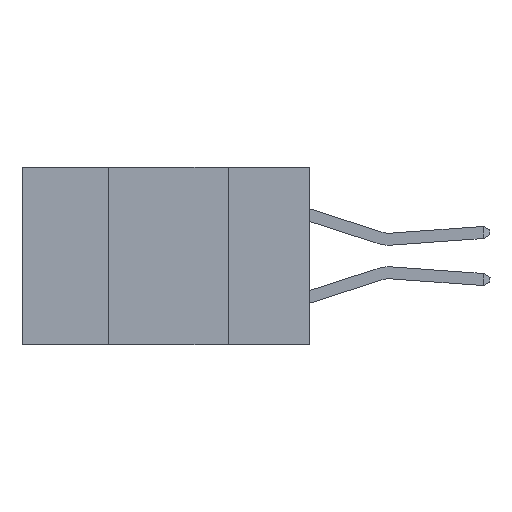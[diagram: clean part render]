
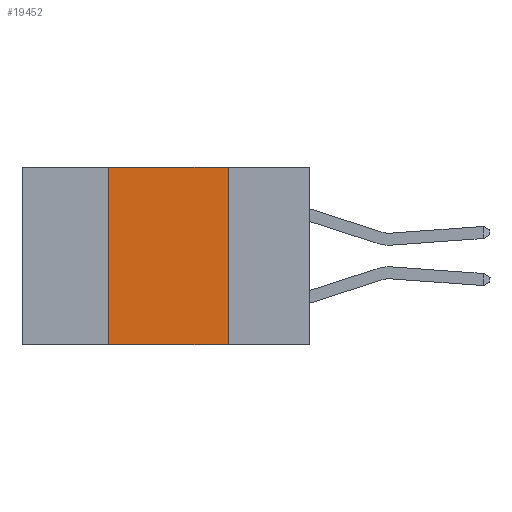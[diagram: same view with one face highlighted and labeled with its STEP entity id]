
A CAD part, left-side view. The second image highlights one B-rep face of the part: STEP entity #19452.
In plain terms, the highlighted planar face has unit normal (-1, 0, 0).
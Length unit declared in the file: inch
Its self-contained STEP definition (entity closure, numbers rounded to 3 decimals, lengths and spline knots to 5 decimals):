
#241 = FACE_OUTER_BOUND ( 'NONE', #21795, .T. ) ;
#1564 = EDGE_CURVE ( 'NONE', #21001, #3537, #8255, .T. ) ;
#2190 = DIRECTION ( 'NONE',  ( 0., -1., 0. ) ) ;
#2445 = DIRECTION ( 'NONE',  ( 0., 0., 1. ) ) ;
#2733 = CARTESIAN_POINT ( 'NONE',  ( 0., 0.42, -0.37 ) ) ;
#2795 = CARTESIAN_POINT ( 'NONE',  ( 0., 0.6, -0.37 ) ) ;
#2815 = EDGE_CURVE ( 'NONE', #21001, #21467, #16242, .T. ) ;
#2859 = VECTOR ( 'NONE', #2190, 39.37008 ) ;
#3138 = ORIENTED_EDGE ( 'NONE', *, *, #5326, .F. ) ;
#3297 = ORIENTED_EDGE ( 'NONE', *, *, #7728, .F. ) ;
#3537 = VERTEX_POINT ( 'NONE', #6032 ) ;
#3904 = ORIENTED_EDGE ( 'NONE', *, *, #2815, .F. ) ;
#4496 = CARTESIAN_POINT ( 'NONE',  ( 0., 0.17, 0. ) ) ;
#5256 = ORIENTED_EDGE ( 'NONE', *, *, #1564, .T. ) ;
#5326 = EDGE_CURVE ( 'NONE', #21467, #21149, #6449, .T. ) ;
#5560 = CARTESIAN_POINT ( 'NONE',  ( 0., 0.6, 0. ) ) ;
#6032 = CARTESIAN_POINT ( 'NONE',  ( 0., 0.17, -0.37 ) ) ;
#6037 = CARTESIAN_POINT ( 'NONE',  ( 0., 0.6, 0. ) ) ;
#6449 = LINE ( 'NONE', #6037, #15602 ) ;
#6546 = VECTOR ( 'NONE', #8542, 39.37008 ) ;
#7112 = VECTOR ( 'NONE', #2445, 39.37008 ) ;
#7728 = EDGE_CURVE ( 'NONE', #21149, #3537, #15163, .T. ) ;
#7798 = DIRECTION ( 'NONE',  ( 0., -1., 0. ) ) ;
#8255 = LINE ( 'NONE', #2795, #2859 ) ;
#8542 = DIRECTION ( 'NONE',  ( 0., 0., -1. ) ) ;
#8870 = CARTESIAN_POINT ( 'NONE',  ( 0., 0.42, 0. ) ) ;
#9098 = DIRECTION ( 'NONE',  ( 1., 0., 0. ) ) ;
#9883 = AXIS2_PLACEMENT_3D ( 'NONE', #5560, #9098, #21088 ) ;
#14184 = PLANE ( 'NONE',  #9883 ) ;
#15163 = LINE ( 'NONE', #18816, #6546 ) ;
#15602 = VECTOR ( 'NONE', #7798, 39.37008 ) ;
#16242 = LINE ( 'NONE', #2733, #7112 ) ;
#16385 = CARTESIAN_POINT ( 'NONE',  ( 0., 0.42, -0.37 ) ) ;
#18816 = CARTESIAN_POINT ( 'NONE',  ( 0., 0.17, -0.37 ) ) ;
#19452 = ADVANCED_FACE ( 'NONE', ( #241 ), #14184, .F. ) ;
#21001 = VERTEX_POINT ( 'NONE', #16385 ) ;
#21088 = DIRECTION ( 'NONE',  ( 0., 0., -1. ) ) ;
#21149 = VERTEX_POINT ( 'NONE', #4496 ) ;
#21467 = VERTEX_POINT ( 'NONE', #8870 ) ;
#21795 = EDGE_LOOP ( 'NONE', ( #3297, #3138, #3904, #5256 ) ) ;
